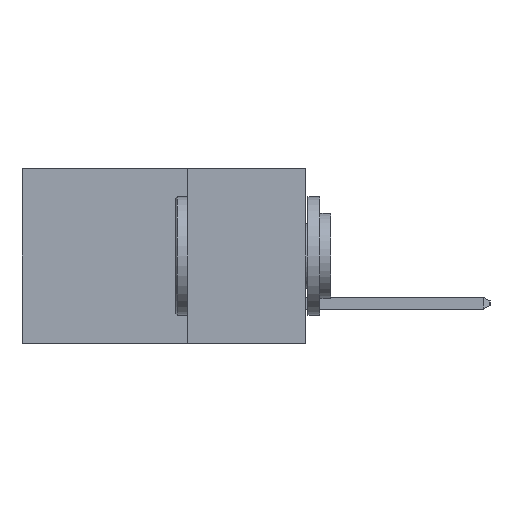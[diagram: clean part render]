
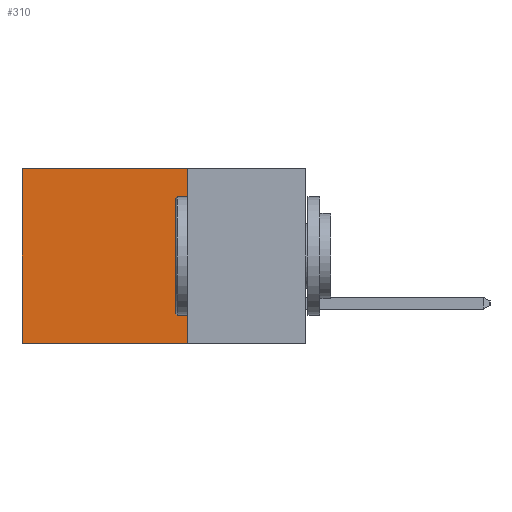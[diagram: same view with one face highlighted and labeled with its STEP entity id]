
A CAD part, left-side view. The second image highlights one B-rep face of the part: STEP entity #310.
In plain terms, the highlighted planar face has unit normal (-1, 0, 0).
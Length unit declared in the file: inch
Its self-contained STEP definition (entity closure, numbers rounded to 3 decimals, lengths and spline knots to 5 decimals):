
#310 = ADVANCED_FACE ( 'NONE', ( #5951 ), #4116, .F. ) ;
#337 = DIRECTION ( 'NONE',  ( 0., 0., -1. ) ) ;
#572 = EDGE_LOOP ( 'NONE', ( #674, #1896, #7428, #11413 ) ) ;
#674 = ORIENTED_EDGE ( 'NONE', *, *, #897, .T. ) ;
#897 = EDGE_CURVE ( 'NONE', #4793, #8676, #10804, .T. ) ;
#1167 = LINE ( 'NONE', #6714, #8740 ) ;
#1238 = VERTEX_POINT ( 'NONE', #4357 ) ;
#1723 = VECTOR ( 'NONE', #7383, 39.37008 ) ;
#1896 = ORIENTED_EDGE ( 'NONE', *, *, #4551, .F. ) ;
#2181 = EDGE_CURVE ( 'NONE', #1238, #4793, #1167, .T. ) ;
#2291 = DIRECTION ( 'NONE',  ( 1., 0., 0. ) ) ;
#2614 = DIRECTION ( 'NONE',  ( 0., 0., -1. ) ) ;
#3030 = CARTESIAN_POINT ( 'NONE',  ( 0.298, 0.25, 0. ) ) ;
#3569 = CARTESIAN_POINT ( 'NONE',  ( 0.298, 0.6, 0. ) ) ;
#4116 = PLANE ( 'NONE',  #8927 ) ;
#4203 = LINE ( 'NONE', #8303, #1723 ) ;
#4357 = CARTESIAN_POINT ( 'NONE',  ( 0.298, 0.25, 0. ) ) ;
#4551 = EDGE_CURVE ( 'NONE', #6617, #8676, #11064, .T. ) ;
#4793 = VERTEX_POINT ( 'NONE', #9852 ) ;
#5432 = EDGE_CURVE ( 'NONE', #1238, #6617, #4203, .T. ) ;
#5447 = CARTESIAN_POINT ( 'NONE',  ( 0.298, 0.25, -0.37 ) ) ;
#5951 = FACE_OUTER_BOUND ( 'NONE', #572, .T. ) ;
#6617 = VERTEX_POINT ( 'NONE', #5447 ) ;
#6714 = CARTESIAN_POINT ( 'NONE',  ( 0.298, 0.25, 0. ) ) ;
#7383 = DIRECTION ( 'NONE',  ( 0., 0., -1. ) ) ;
#7428 = ORIENTED_EDGE ( 'NONE', *, *, #5432, .F. ) ;
#8202 = VECTOR ( 'NONE', #2614, 39.37008 ) ;
#8303 = CARTESIAN_POINT ( 'NONE',  ( 0.298, 0.25, 0. ) ) ;
#8676 = VERTEX_POINT ( 'NONE', #9681 ) ;
#8740 = VECTOR ( 'NONE', #10580, 39.37008 ) ;
#8745 = VECTOR ( 'NONE', #11175, 39.37008 ) ;
#8927 = AXIS2_PLACEMENT_3D ( 'NONE', #3030, #2291, #337 ) ;
#9681 = CARTESIAN_POINT ( 'NONE',  ( 0.298, 0.6, -0.37 ) ) ;
#9852 = CARTESIAN_POINT ( 'NONE',  ( 0.298, 0.6, 0. ) ) ;
#10580 = DIRECTION ( 'NONE',  ( 0., 1., 0. ) ) ;
#10804 = LINE ( 'NONE', #3569, #8202 ) ;
#11064 = LINE ( 'NONE', #11359, #8745 ) ;
#11175 = DIRECTION ( 'NONE',  ( 0., 1., 0. ) ) ;
#11359 = CARTESIAN_POINT ( 'NONE',  ( 0.298, 0.25, -0.37 ) ) ;
#11413 = ORIENTED_EDGE ( 'NONE', *, *, #2181, .T. ) ;
